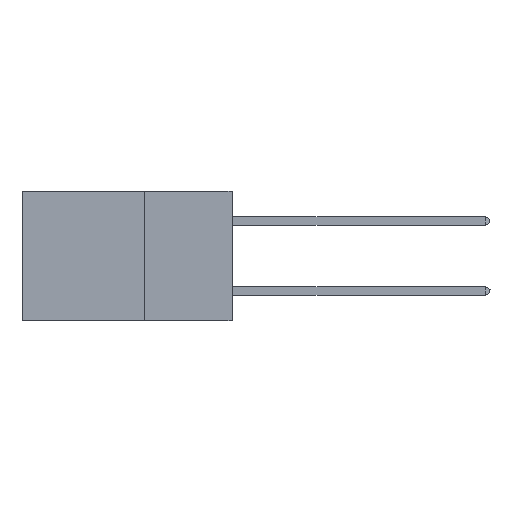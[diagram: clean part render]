
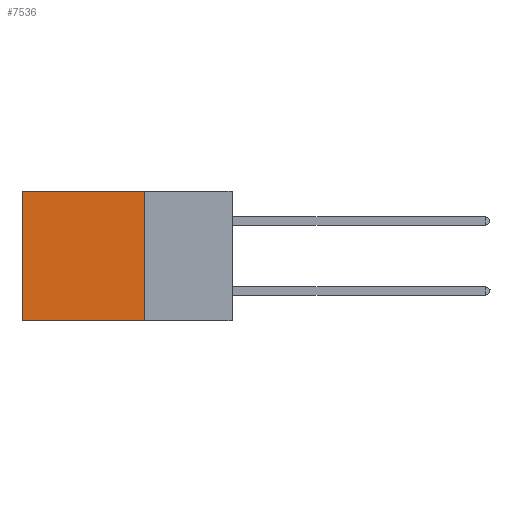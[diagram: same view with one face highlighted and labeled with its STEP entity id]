
A CAD part, left-side view. The second image highlights one B-rep face of the part: STEP entity #7536.
In plain terms, the highlighted planar face has unit normal (-1, 0, 0).
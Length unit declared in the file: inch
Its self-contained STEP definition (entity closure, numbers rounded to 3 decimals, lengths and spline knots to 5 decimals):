
#1197 = LINE ( 'NONE', #10571, #12333 ) ;
#1843 = EDGE_LOOP ( 'NONE', ( #2172, #3505, #8196, #12613 ) ) ;
#2172 = ORIENTED_EDGE ( 'NONE', *, *, #11113, .T. ) ;
#3505 = ORIENTED_EDGE ( 'NONE', *, *, #8318, .F. ) ;
#3702 = LINE ( 'NONE', #16161, #9830 ) ;
#4087 = EDGE_CURVE ( 'NONE', #14334, #14582, #1197, .T. ) ;
#4667 = PLANE ( 'NONE',  #17838 ) ;
#4860 = DIRECTION ( 'NONE',  ( 0., 1., 0. ) ) ;
#5043 = DIRECTION ( 'NONE',  ( 0., 0., -1. ) ) ;
#5474 = LINE ( 'NONE', #6909, #5673 ) ;
#5673 = VECTOR ( 'NONE', #12533, 39.37008 ) ;
#6609 = CARTESIAN_POINT ( 'NONE',  ( 0.2875, 0.25, -0.37 ) ) ;
#6742 = CARTESIAN_POINT ( 'NONE',  ( 0.2875, 0.25, 0. ) ) ;
#6909 = CARTESIAN_POINT ( 'NONE',  ( 0.2875, 0.25, 0. ) ) ;
#7119 = VERTEX_POINT ( 'NONE', #6609 ) ;
#7319 = EDGE_CURVE ( 'NONE', #14334, #7119, #5474, .T. ) ;
#7536 = ADVANCED_FACE ( 'NONE', ( #13716 ), #4667, .F. ) ;
#8196 = ORIENTED_EDGE ( 'NONE', *, *, #7319, .F. ) ;
#8318 = EDGE_CURVE ( 'NONE', #7119, #15494, #3702, .T. ) ;
#9072 = VECTOR ( 'NONE', #5043, 39.37008 ) ;
#9830 = VECTOR ( 'NONE', #4860, 39.37008 ) ;
#10571 = CARTESIAN_POINT ( 'NONE',  ( 0.2875, 0.25, 0. ) ) ;
#10634 = DIRECTION ( 'NONE',  ( 0., 1., 0. ) ) ;
#10775 = CARTESIAN_POINT ( 'NONE',  ( 0.2875, 0.6, 0. ) ) ;
#11113 = EDGE_CURVE ( 'NONE', #14582, #15494, #15991, .T. ) ;
#11654 = CARTESIAN_POINT ( 'NONE',  ( 0.2875, 0.25, 0. ) ) ;
#12333 = VECTOR ( 'NONE', #10634, 39.37008 ) ;
#12533 = DIRECTION ( 'NONE',  ( 0., 0., -1. ) ) ;
#12613 = ORIENTED_EDGE ( 'NONE', *, *, #4087, .T. ) ;
#13051 = DIRECTION ( 'NONE',  ( 1., 0., 0. ) ) ;
#13716 = FACE_OUTER_BOUND ( 'NONE', #1843, .T. ) ;
#13790 = CARTESIAN_POINT ( 'NONE',  ( 0.2875, 0.6, 0. ) ) ;
#14334 = VERTEX_POINT ( 'NONE', #6742 ) ;
#14582 = VERTEX_POINT ( 'NONE', #13790 ) ;
#14712 = CARTESIAN_POINT ( 'NONE',  ( 0.2875, 0.6, -0.37 ) ) ;
#15494 = VERTEX_POINT ( 'NONE', #14712 ) ;
#15730 = DIRECTION ( 'NONE',  ( 0., 0., -1. ) ) ;
#15991 = LINE ( 'NONE', #10775, #9072 ) ;
#16161 = CARTESIAN_POINT ( 'NONE',  ( 0.2875, 0.25, -0.37 ) ) ;
#17838 = AXIS2_PLACEMENT_3D ( 'NONE', #11654, #13051, #15730 ) ;
